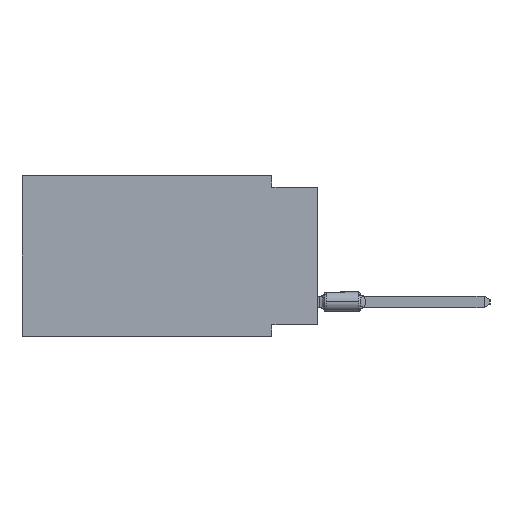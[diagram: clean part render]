
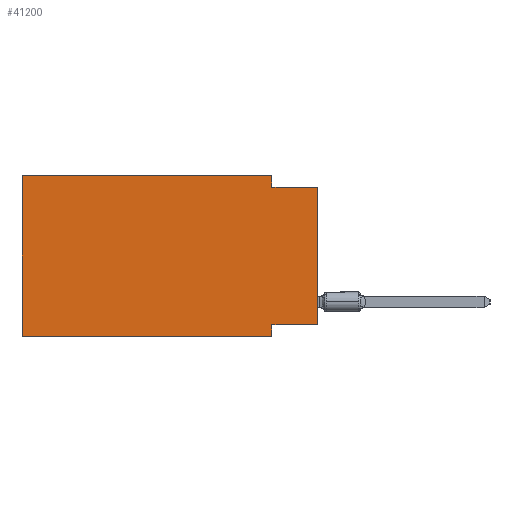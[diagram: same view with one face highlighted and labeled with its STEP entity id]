
A CAD part, left-side view. The second image highlights one B-rep face of the part: STEP entity #41200.
In plain terms, the highlighted planar face has unit normal (-1, 0, 0).
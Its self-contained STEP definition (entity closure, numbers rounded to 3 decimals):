
#1097 = CARTESIAN_POINT ( 'NONE',  ( 0., 0., -8.255 ) ) ;
#1225 = LINE ( 'NONE', #16608, #13824 ) ;
#1743 = CARTESIAN_POINT ( 'NONE',  ( 0., 16.383, -8.89 ) ) ;
#2633 = VECTOR ( 'NONE', #55223, 1000. ) ;
#3198 = ORIENTED_EDGE ( 'NONE', *, *, #41471, .F. ) ;
#3589 = LINE ( 'NONE', #19633, #55627 ) ;
#4305 = VECTOR ( 'NONE', #47721, 1000. ) ;
#5124 = ORIENTED_EDGE ( 'NONE', *, *, #55092, .T. ) ;
#5668 = FACE_OUTER_BOUND ( 'NONE', #42635, .T. ) ;
#7516 = LINE ( 'NONE', #1743, #21536 ) ;
#11275 = VECTOR ( 'NONE', #39627, 1000. ) ;
#12326 = DIRECTION ( 'NONE',  ( 0., -1., 0. ) ) ;
#13824 = VECTOR ( 'NONE', #37470, 1000. ) ;
#13863 = LINE ( 'NONE', #50763, #2633 ) ;
#16015 = CARTESIAN_POINT ( 'NONE',  ( 0., 16.383, 0. ) ) ;
#16273 = LINE ( 'NONE', #37481, #4305 ) ;
#16608 = CARTESIAN_POINT ( 'NONE',  ( 0., 2.54, 0. ) ) ;
#17273 = ORIENTED_EDGE ( 'NONE', *, *, #22786, .F. ) ;
#17608 = EDGE_CURVE ( 'NONE', #52112, #44532, #1225, .T. ) ;
#18654 = EDGE_CURVE ( 'NONE', #23552, #41520, #7516, .T. ) ;
#19633 = CARTESIAN_POINT ( 'NONE',  ( 0., 0., -0.635 ) ) ;
#20655 = CARTESIAN_POINT ( 'NONE',  ( 0., 16.383, 0. ) ) ;
#21536 = VECTOR ( 'NONE', #12326, 1000. ) ;
#21614 = VERTEX_POINT ( 'NONE', #50456 ) ;
#22074 = ORIENTED_EDGE ( 'NONE', *, *, #17608, .F. ) ;
#22786 = EDGE_CURVE ( 'NONE', #62383, #41520, #16273, .T. ) ;
#23552 = VERTEX_POINT ( 'NONE', #25008 ) ;
#24577 = LINE ( 'NONE', #30706, #11275 ) ;
#25008 = CARTESIAN_POINT ( 'NONE',  ( 0., 16.383, -8.89 ) ) ;
#26525 = PLANE ( 'NONE',  #54542 ) ;
#30578 = VECTOR ( 'NONE', #61495, 1000. ) ;
#30706 = CARTESIAN_POINT ( 'NONE',  ( 0., 16.383, 0. ) ) ;
#31371 = EDGE_CURVE ( 'NONE', #45966, #62383, #39292, .T. ) ;
#32970 = ORIENTED_EDGE ( 'NONE', *, *, #64452, .F. ) ;
#34664 = ORIENTED_EDGE ( 'NONE', *, *, #18654, .T. ) ;
#37234 = EDGE_CURVE ( 'NONE', #23552, #49850, #24577, .T. ) ;
#37470 = DIRECTION ( 'NONE',  ( 0., 0., -1. ) ) ;
#37481 = CARTESIAN_POINT ( 'NONE',  ( 0., 2.54, -8.89 ) ) ;
#39131 = CARTESIAN_POINT ( 'NONE',  ( 0., 2.54, 0. ) ) ;
#39292 = LINE ( 'NONE', #64951, #56100 ) ;
#39627 = DIRECTION ( 'NONE',  ( 0., 0., 1. ) ) ;
#41200 = ADVANCED_FACE ( 'NONE', ( #5668 ), #26525, .F. ) ;
#41471 = EDGE_CURVE ( 'NONE', #44532, #21614, #3589, .T. ) ;
#41520 = VERTEX_POINT ( 'NONE', #57875 ) ;
#42635 = EDGE_LOOP ( 'NONE', ( #5124, #3198, #22074, #32970, #60853, #34664, #17273, #55139 ) ) ;
#44210 = CARTESIAN_POINT ( 'NONE',  ( 0., 2.54, -0.635 ) ) ;
#44532 = VERTEX_POINT ( 'NONE', #44210 ) ;
#45135 = CARTESIAN_POINT ( 'NONE',  ( 0., 2.54, -8.255 ) ) ;
#45966 = VERTEX_POINT ( 'NONE', #1097 ) ;
#47376 = CARTESIAN_POINT ( 'NONE',  ( 0., 16.383, 0. ) ) ;
#47721 = DIRECTION ( 'NONE',  ( 0., 0., -1. ) ) ;
#49850 = VERTEX_POINT ( 'NONE', #20655 ) ;
#50456 = CARTESIAN_POINT ( 'NONE',  ( 0., 0., -0.635 ) ) ;
#50763 = CARTESIAN_POINT ( 'NONE',  ( 0., 0., 0. ) ) ;
#52112 = VERTEX_POINT ( 'NONE', #39131 ) ;
#53515 = DIRECTION ( 'NONE',  ( 0., 0., -1. ) ) ;
#54542 = AXIS2_PLACEMENT_3D ( 'NONE', #47376, #58321, #53515 ) ;
#55092 = EDGE_CURVE ( 'NONE', #45966, #21614, #13863, .T. ) ;
#55139 = ORIENTED_EDGE ( 'NONE', *, *, #31371, .F. ) ;
#55223 = DIRECTION ( 'NONE',  ( 0., 0., 1. ) ) ;
#55627 = VECTOR ( 'NONE', #61327, 1000. ) ;
#56100 = VECTOR ( 'NONE', #60131, 1000. ) ;
#57875 = CARTESIAN_POINT ( 'NONE',  ( 0., 2.54, -8.89 ) ) ;
#58321 = DIRECTION ( 'NONE',  ( 1., 0., 0. ) ) ;
#60131 = DIRECTION ( 'NONE',  ( 0., 1., 0. ) ) ;
#60853 = ORIENTED_EDGE ( 'NONE', *, *, #37234, .F. ) ;
#61327 = DIRECTION ( 'NONE',  ( 0., -1., 0. ) ) ;
#61495 = DIRECTION ( 'NONE',  ( 0., -1., 0. ) ) ;
#62383 = VERTEX_POINT ( 'NONE', #45135 ) ;
#62843 = LINE ( 'NONE', #16015, #30578 ) ;
#64452 = EDGE_CURVE ( 'NONE', #49850, #52112, #62843, .T. ) ;
#64951 = CARTESIAN_POINT ( 'NONE',  ( 0., 0., -8.255 ) ) ;
